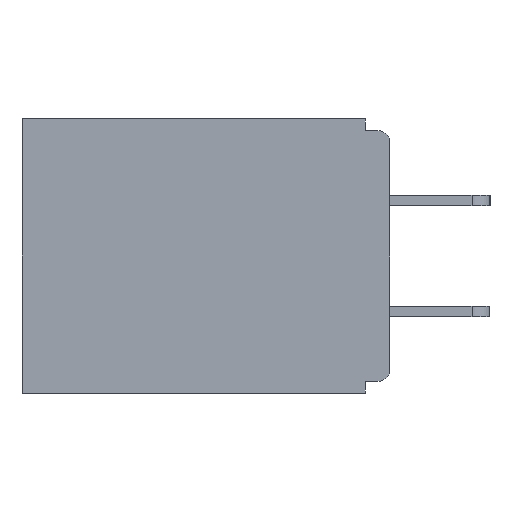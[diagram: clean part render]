
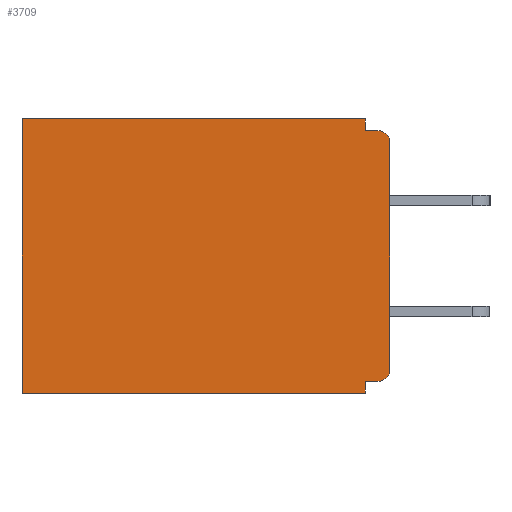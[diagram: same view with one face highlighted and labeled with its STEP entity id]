
A CAD part, left-side view. The second image highlights one B-rep face of the part: STEP entity #3709.
In plain terms, the highlighted planar face has unit normal (-1, 0, 0).
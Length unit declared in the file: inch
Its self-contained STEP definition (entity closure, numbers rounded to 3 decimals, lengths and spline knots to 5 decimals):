
#27 = CARTESIAN_POINT ( 'NONE',  ( 0.298, 0.031, -0.343 ) ) ;
#233 = CARTESIAN_POINT ( 'NONE',  ( 0.298, 0., 0. ) ) ;
#705 = LINE ( 'NONE', #7695, #3329 ) ;
#771 = LINE ( 'NONE', #3888, #5349 ) ;
#827 = DIRECTION ( 'NONE',  ( 1., 0., 0. ) ) ;
#1252 = VERTEX_POINT ( 'NONE', #5441 ) ;
#1545 = CARTESIAN_POINT ( 'NONE',  ( 0.298, 0.46, 0. ) ) ;
#1709 = VECTOR ( 'NONE', #10371, 39.37008 ) ;
#1772 = CARTESIAN_POINT ( 'NONE',  ( 0.298, 0.031, -0.328 ) ) ;
#1798 = CARTESIAN_POINT ( 'NONE',  ( 0.298, 0.031, -0.343 ) ) ;
#1807 = EDGE_CURVE ( 'NONE', #1252, #6300, #2739, .T. ) ;
#1814 = DIRECTION ( 'NONE',  ( -1., 0., 0. ) ) ;
#1928 = VERTEX_POINT ( 'NONE', #1772 ) ;
#2009 = LINE ( 'NONE', #1798, #5602 ) ;
#2270 = VERTEX_POINT ( 'NONE', #7173 ) ;
#2338 = AXIS2_PLACEMENT_3D ( 'NONE', #11322, #827, #10363 ) ;
#2357 = LINE ( 'NONE', #233, #5421 ) ;
#2374 = DIRECTION ( 'NONE',  ( 0., 1., 0. ) ) ;
#2423 = CARTESIAN_POINT ( 'NONE',  ( 0.298, 0.015, -0.03 ) ) ;
#2512 = LINE ( 'NONE', #7841, #1709 ) ;
#2739 = LINE ( 'NONE', #6791, #4413 ) ;
#3065 = CIRCLE ( 'NONE', #4858, 0.015 ) ;
#3235 = EDGE_CURVE ( 'NONE', #1252, #5463, #2009, .T. ) ;
#3237 = EDGE_CURVE ( 'NONE', #1928, #8649, #8232, .T. ) ;
#3322 = EDGE_CURVE ( 'NONE', #9767, #1928, #771, .T. ) ;
#3329 = VECTOR ( 'NONE', #10303, 39.37008 ) ;
#3519 = DIRECTION ( 'NONE',  ( 0., 0., -1. ) ) ;
#3647 = VERTEX_POINT ( 'NONE', #7436 ) ;
#3654 = ORIENTED_EDGE ( 'NONE', *, *, #3237, .F. ) ;
#3709 = ADVANCED_FACE ( 'NONE', ( #8535 ), #4126, .F. ) ;
#3888 = CARTESIAN_POINT ( 'NONE',  ( 0.298, 0., -0.328 ) ) ;
#4126 = PLANE ( 'NONE',  #2338 ) ;
#4200 = ORIENTED_EDGE ( 'NONE', *, *, #3322, .F. ) ;
#4413 = VECTOR ( 'NONE', #2374, 39.37008 ) ;
#4488 = AXIS2_PLACEMENT_3D ( 'NONE', #6754, #11152, #8543 ) ;
#4804 = ORIENTED_EDGE ( 'NONE', *, *, #8497, .F. ) ;
#4858 = AXIS2_PLACEMENT_3D ( 'NONE', #2423, #1814, #3519 ) ;
#5349 = VECTOR ( 'NONE', #8167, 39.37008 ) ;
#5367 = ORIENTED_EDGE ( 'NONE', *, *, #1807, .T. ) ;
#5421 = VECTOR ( 'NONE', #10782, 39.37008 ) ;
#5441 = CARTESIAN_POINT ( 'NONE',  ( 0.298, 0.031, 0. ) ) ;
#5463 = VERTEX_POINT ( 'NONE', #8541 ) ;
#5497 = EDGE_CURVE ( 'NONE', #5463, #7720, #2512, .T. ) ;
#5602 = VECTOR ( 'NONE', #8092, 39.37008 ) ;
#5839 = EDGE_CURVE ( 'NONE', #2270, #7720, #3065, .T. ) ;
#5885 = CARTESIAN_POINT ( 'NONE',  ( 0.298, 0., -0.343 ) ) ;
#6300 = VERTEX_POINT ( 'NONE', #1545 ) ;
#6400 = CARTESIAN_POINT ( 'NONE',  ( 0.298, 0.46, -0.343 ) ) ;
#6565 = EDGE_CURVE ( 'NONE', #8649, #8522, #9368, .T. ) ;
#6732 = ORIENTED_EDGE ( 'NONE', *, *, #3235, .F. ) ;
#6754 = CARTESIAN_POINT ( 'NONE',  ( 0.298, 0.015, -0.313 ) ) ;
#6791 = CARTESIAN_POINT ( 'NONE',  ( 0.298, 0., 0. ) ) ;
#7173 = CARTESIAN_POINT ( 'NONE',  ( 0.298, 0., -0.03 ) ) ;
#7395 = EDGE_LOOP ( 'NONE', ( #10424, #10210, #6732, #5367, #9885, #7967, #3654, #4200, #9798, #4804 ) ) ;
#7436 = CARTESIAN_POINT ( 'NONE',  ( 0.298, 0., -0.313 ) ) ;
#7689 = VECTOR ( 'NONE', #8049, 39.37008 ) ;
#7695 = CARTESIAN_POINT ( 'NONE',  ( 0.298, 0.46, 0. ) ) ;
#7720 = VERTEX_POINT ( 'NONE', #10145 ) ;
#7755 = EDGE_CURVE ( 'NONE', #9767, #3647, #10664, .T. ) ;
#7841 = CARTESIAN_POINT ( 'NONE',  ( 0.298, 0., -0.015 ) ) ;
#7873 = VECTOR ( 'NONE', #9468, 39.37008 ) ;
#7967 = ORIENTED_EDGE ( 'NONE', *, *, #6565, .F. ) ;
#8049 = DIRECTION ( 'NONE',  ( 0., 0., -1. ) ) ;
#8092 = DIRECTION ( 'NONE',  ( 0., 0., -1. ) ) ;
#8167 = DIRECTION ( 'NONE',  ( 0., 1., 0. ) ) ;
#8232 = LINE ( 'NONE', #27, #7689 ) ;
#8435 = CARTESIAN_POINT ( 'NONE',  ( 0.298, 0.031, -0.343 ) ) ;
#8497 = EDGE_CURVE ( 'NONE', #2270, #3647, #2357, .T. ) ;
#8522 = VERTEX_POINT ( 'NONE', #6400 ) ;
#8535 = FACE_OUTER_BOUND ( 'NONE', #7395, .T. ) ;
#8541 = CARTESIAN_POINT ( 'NONE',  ( 0.298, 0.031, -0.015 ) ) ;
#8543 = DIRECTION ( 'NONE',  ( 0., 0., -1. ) ) ;
#8632 = EDGE_CURVE ( 'NONE', #6300, #8522, #705, .T. ) ;
#8649 = VERTEX_POINT ( 'NONE', #8435 ) ;
#9368 = LINE ( 'NONE', #5885, #7873 ) ;
#9468 = DIRECTION ( 'NONE',  ( 0., 1., 0. ) ) ;
#9767 = VERTEX_POINT ( 'NONE', #10649 ) ;
#9798 = ORIENTED_EDGE ( 'NONE', *, *, #7755, .T. ) ;
#9885 = ORIENTED_EDGE ( 'NONE', *, *, #8632, .T. ) ;
#10145 = CARTESIAN_POINT ( 'NONE',  ( 0.298, 0.015, -0.015 ) ) ;
#10210 = ORIENTED_EDGE ( 'NONE', *, *, #5497, .F. ) ;
#10303 = DIRECTION ( 'NONE',  ( 0., 0., -1. ) ) ;
#10363 = DIRECTION ( 'NONE',  ( 0., 0., -1. ) ) ;
#10371 = DIRECTION ( 'NONE',  ( 0., -1., 0. ) ) ;
#10424 = ORIENTED_EDGE ( 'NONE', *, *, #5839, .T. ) ;
#10649 = CARTESIAN_POINT ( 'NONE',  ( 0.298, 0.015, -0.328 ) ) ;
#10664 = CIRCLE ( 'NONE', #4488, 0.015 ) ;
#10782 = DIRECTION ( 'NONE',  ( 0., 0., -1. ) ) ;
#11152 = DIRECTION ( 'NONE',  ( -1., 0., 0. ) ) ;
#11322 = CARTESIAN_POINT ( 'NONE',  ( 0.298, 0., 0. ) ) ;
